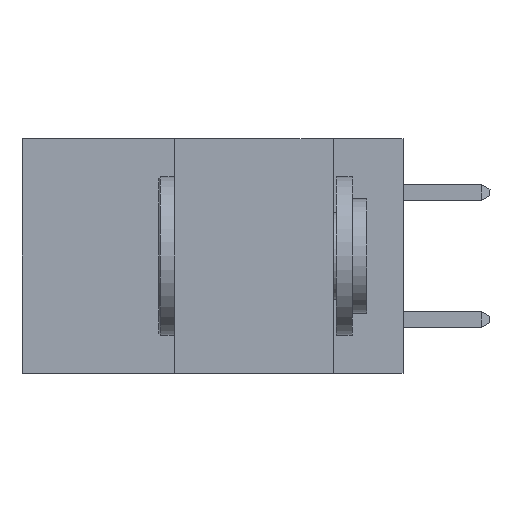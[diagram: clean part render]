
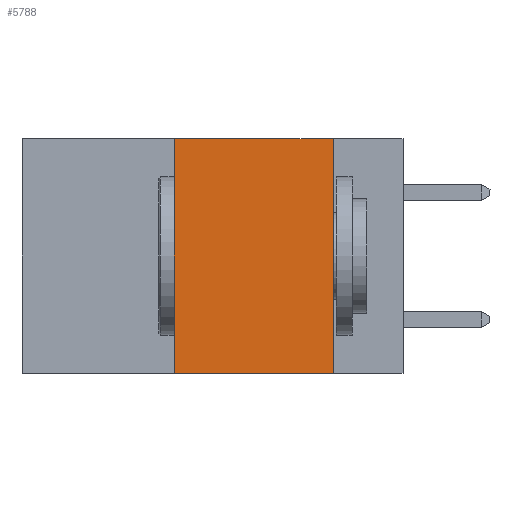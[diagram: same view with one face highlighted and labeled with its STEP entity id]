
A CAD part, left-side view. The second image highlights one B-rep face of the part: STEP entity #5788.
In plain terms, the highlighted planar face has unit normal (-1, 0, 0).
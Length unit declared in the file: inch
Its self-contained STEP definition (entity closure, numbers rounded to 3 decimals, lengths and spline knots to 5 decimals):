
#67 = DIRECTION ( 'NONE',  ( 1., 0., 0. ) ) ;
#82 = PLANE ( 'NONE',  #6514 ) ;
#268 = LINE ( 'NONE', #8882, #621 ) ;
#341 = DIRECTION ( 'NONE',  ( 0., -1., 0. ) ) ;
#380 = VERTEX_POINT ( 'NONE', #8144 ) ;
#573 = CARTESIAN_POINT ( 'NONE',  ( 0., 0.6, -0.37 ) ) ;
#621 = VECTOR ( 'NONE', #1327, 39.37008 ) ;
#1001 = VERTEX_POINT ( 'NONE', #6827 ) ;
#1005 = VERTEX_POINT ( 'NONE', #6676 ) ;
#1206 = VERTEX_POINT ( 'NONE', #5016 ) ;
#1294 = ORIENTED_EDGE ( 'NONE', *, *, #10724, .F. ) ;
#1327 = DIRECTION ( 'NONE',  ( 0., 0., -1. ) ) ;
#1347 = ORIENTED_EDGE ( 'NONE', *, *, #6199, .F. ) ;
#1411 = ORIENTED_EDGE ( 'NONE', *, *, #4101, .F. ) ;
#1456 = EDGE_CURVE ( 'NONE', #1206, #1001, #2362, .T. ) ;
#1584 = ORIENTED_EDGE ( 'NONE', *, *, #1456, .T. ) ;
#2362 = LINE ( 'NONE', #573, #8708 ) ;
#4101 = EDGE_CURVE ( 'NONE', #1206, #380, #8775, .T. ) ;
#5016 = CARTESIAN_POINT ( 'NONE',  ( 0., 0.36, -0.37 ) ) ;
#5425 = LINE ( 'NONE', #7173, #7259 ) ;
#5788 = ADVANCED_FACE ( 'NONE', ( #9100 ), #82, .F. ) ;
#6199 = EDGE_CURVE ( 'NONE', #380, #1005, #5425, .T. ) ;
#6514 = AXIS2_PLACEMENT_3D ( 'NONE', #9185, #67, #11027 ) ;
#6676 = CARTESIAN_POINT ( 'NONE',  ( 0., 0.11, 0. ) ) ;
#6827 = CARTESIAN_POINT ( 'NONE',  ( 0., 0.11, -0.37 ) ) ;
#7139 = DIRECTION ( 'NONE',  ( 0., -1., 0. ) ) ;
#7173 = CARTESIAN_POINT ( 'NONE',  ( 0., 0.6, 0. ) ) ;
#7259 = VECTOR ( 'NONE', #7139, 39.37008 ) ;
#8095 = EDGE_LOOP ( 'NONE', ( #1294, #1347, #1411, #1584 ) ) ;
#8144 = CARTESIAN_POINT ( 'NONE',  ( 0., 0.36, 0. ) ) ;
#8708 = VECTOR ( 'NONE', #341, 39.37008 ) ;
#8775 = LINE ( 'NONE', #10367, #10610 ) ;
#8882 = CARTESIAN_POINT ( 'NONE',  ( 0., 0.11, 0. ) ) ;
#9100 = FACE_OUTER_BOUND ( 'NONE', #8095, .T. ) ;
#9185 = CARTESIAN_POINT ( 'NONE',  ( 0., 0.6, 0. ) ) ;
#10354 = DIRECTION ( 'NONE',  ( 0., 0., 1. ) ) ;
#10367 = CARTESIAN_POINT ( 'NONE',  ( 0., 0.36, 0. ) ) ;
#10610 = VECTOR ( 'NONE', #10354, 39.37008 ) ;
#10724 = EDGE_CURVE ( 'NONE', #1005, #1001, #268, .T. ) ;
#11027 = DIRECTION ( 'NONE',  ( 0., 0., -1. ) ) ;
